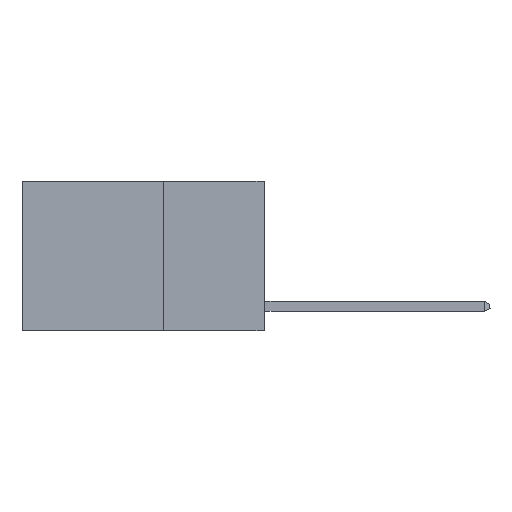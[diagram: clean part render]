
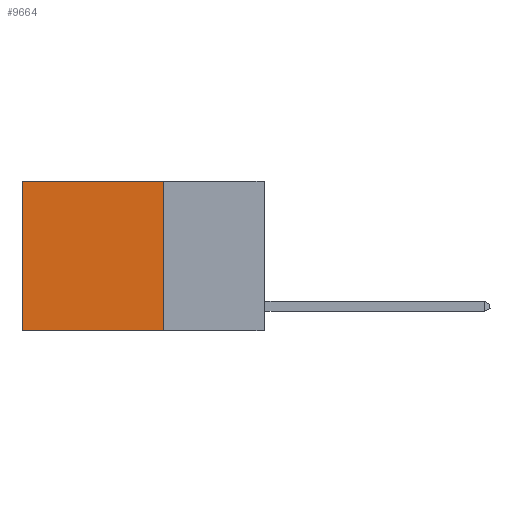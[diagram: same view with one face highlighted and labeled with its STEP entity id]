
A CAD part, left-side view. The second image highlights one B-rep face of the part: STEP entity #9664.
In plain terms, the highlighted planar face has unit normal (-1, 0, 0).
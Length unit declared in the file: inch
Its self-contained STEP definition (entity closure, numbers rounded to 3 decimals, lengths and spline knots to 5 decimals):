
#146 = EDGE_CURVE ( 'NONE', #2905, #360, #1903, .T. ) ;
#360 = VERTEX_POINT ( 'NONE', #4472 ) ;
#665 = CARTESIAN_POINT ( 'NONE',  ( 0.2625, 0.6, 0. ) ) ;
#823 = DIRECTION ( 'NONE',  ( 0., 0., -1. ) ) ;
#981 = VERTEX_POINT ( 'NONE', #4586 ) ;
#1006 = DIRECTION ( 'NONE',  ( 0., 1., 0. ) ) ;
#1325 = ORIENTED_EDGE ( 'NONE', *, *, #146, .T. ) ;
#1903 = LINE ( 'NONE', #9421, #2906 ) ;
#2809 = VECTOR ( 'NONE', #3079, 39.37008 ) ;
#2905 = VERTEX_POINT ( 'NONE', #665 ) ;
#2906 = VECTOR ( 'NONE', #11390, 39.37008 ) ;
#3079 = DIRECTION ( 'NONE',  ( 0., 0., -1. ) ) ;
#3939 = CARTESIAN_POINT ( 'NONE',  ( 0.2625, 0.25, 0. ) ) ;
#3984 = VECTOR ( 'NONE', #1006, 39.37008 ) ;
#4137 = AXIS2_PLACEMENT_3D ( 'NONE', #8421, #8298, #823 ) ;
#4472 = CARTESIAN_POINT ( 'NONE',  ( 0.2625, 0.6, -0.37 ) ) ;
#4586 = CARTESIAN_POINT ( 'NONE',  ( 0.2625, 0.25, -0.37 ) ) ;
#4611 = EDGE_CURVE ( 'NONE', #981, #360, #9338, .T. ) ;
#6268 = ORIENTED_EDGE ( 'NONE', *, *, #4611, .F. ) ;
#6351 = DIRECTION ( 'NONE',  ( 0., 1., 0. ) ) ;
#6431 = CARTESIAN_POINT ( 'NONE',  ( 0.2625, 0.25, 0. ) ) ;
#7476 = LINE ( 'NONE', #12178, #3984 ) ;
#8034 = VECTOR ( 'NONE', #6351, 39.37008 ) ;
#8083 = ORIENTED_EDGE ( 'NONE', *, *, #11675, .T. ) ;
#8298 = DIRECTION ( 'NONE',  ( 1., 0., 0. ) ) ;
#8421 = CARTESIAN_POINT ( 'NONE',  ( 0.2625, 0.25, 0. ) ) ;
#8505 = EDGE_LOOP ( 'NONE', ( #1325, #6268, #11465, #8083 ) ) ;
#9338 = LINE ( 'NONE', #10127, #8034 ) ;
#9421 = CARTESIAN_POINT ( 'NONE',  ( 0.2625, 0.6, 0. ) ) ;
#9664 = ADVANCED_FACE ( 'NONE', ( #11181 ), #12181, .F. ) ;
#10127 = CARTESIAN_POINT ( 'NONE',  ( 0.2625, 0.25, -0.37 ) ) ;
#10246 = LINE ( 'NONE', #3939, #2809 ) ;
#10920 = VERTEX_POINT ( 'NONE', #6431 ) ;
#11181 = FACE_OUTER_BOUND ( 'NONE', #8505, .T. ) ;
#11280 = EDGE_CURVE ( 'NONE', #10920, #981, #10246, .T. ) ;
#11390 = DIRECTION ( 'NONE',  ( 0., 0., -1. ) ) ;
#11465 = ORIENTED_EDGE ( 'NONE', *, *, #11280, .F. ) ;
#11675 = EDGE_CURVE ( 'NONE', #10920, #2905, #7476, .T. ) ;
#12178 = CARTESIAN_POINT ( 'NONE',  ( 0.2625, 0.25, 0. ) ) ;
#12181 = PLANE ( 'NONE',  #4137 ) ;
